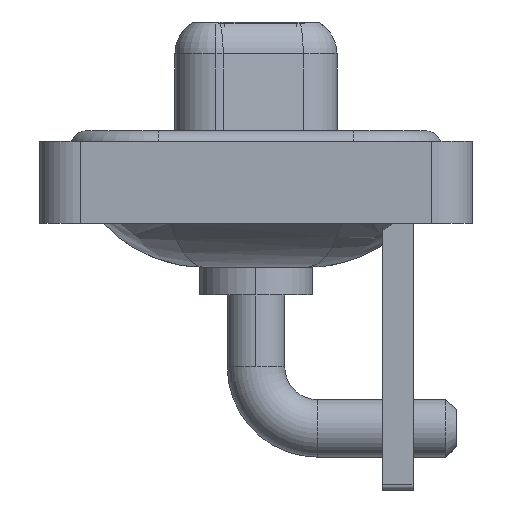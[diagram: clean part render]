
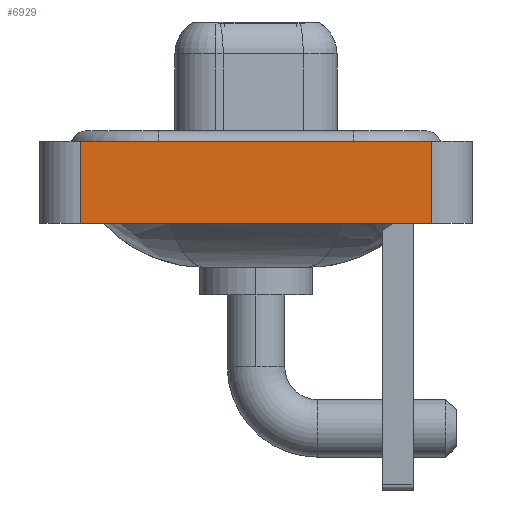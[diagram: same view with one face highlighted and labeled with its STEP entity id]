
A CAD part, left-side view. The second image highlights one B-rep face of the part: STEP entity #6929.
In plain terms, the highlighted planar face has unit normal (-1, 0, 0).
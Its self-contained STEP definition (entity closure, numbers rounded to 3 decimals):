
#339 = PLANE ( 'NONE',  #5335 ) ;
#2868 = DIRECTION ( 'NONE',  ( 0., -1., 0. ) ) ;
#2964 = DIRECTION ( 'NONE',  ( -1., 0., 0. ) ) ;
#3488 = EDGE_CURVE ( 'NONE', #15932, #4345, #7195, .T. ) ;
#4280 = DIRECTION ( 'NONE',  ( 0., 0., 1. ) ) ;
#4345 = VERTEX_POINT ( 'NONE', #6886 ) ;
#5335 = AXIS2_PLACEMENT_3D ( 'NONE', #16402, #2964, #4280 ) ;
#5343 = EDGE_CURVE ( 'NONE', #10010, #9417, #14915, .T. ) ;
#5426 = VECTOR ( 'NONE', #7169, 1000. ) ;
#5608 = CARTESIAN_POINT ( 'NONE',  ( -7.35, -8.55, 0.4 ) ) ;
#6595 = VECTOR ( 'NONE', #15816, 1000. ) ;
#6681 = LINE ( 'NONE', #10476, #6595 ) ;
#6766 = CARTESIAN_POINT ( 'NONE',  ( -7.35, 8.55, -3.6 ) ) ;
#6886 = CARTESIAN_POINT ( 'NONE',  ( -7.35, -8.55, 0.4 ) ) ;
#6903 = LINE ( 'NONE', #10872, #5426 ) ;
#6929 = ADVANCED_FACE ( 'NONE', ( #8513 ), #339, .T. ) ;
#7169 = DIRECTION ( 'NONE',  ( 0., 0., 1. ) ) ;
#7195 = LINE ( 'NONE', #5608, #8643 ) ;
#7876 = ORIENTED_EDGE ( 'NONE', *, *, #8765, .F. ) ;
#8371 = EDGE_LOOP ( 'NONE', ( #15508, #9487, #7876, #15078 ) ) ;
#8513 = FACE_OUTER_BOUND ( 'NONE', #8371, .T. ) ;
#8643 = VECTOR ( 'NONE', #12220, 1000. ) ;
#8765 = EDGE_CURVE ( 'NONE', #10010, #15932, #6903, .T. ) ;
#8960 = CARTESIAN_POINT ( 'NONE',  ( -7.35, -8.55, -3.6 ) ) ;
#9417 = VERTEX_POINT ( 'NONE', #8960 ) ;
#9487 = ORIENTED_EDGE ( 'NONE', *, *, #3488, .F. ) ;
#10010 = VERTEX_POINT ( 'NONE', #6766 ) ;
#10104 = EDGE_CURVE ( 'NONE', #9417, #4345, #6681, .T. ) ;
#10476 = CARTESIAN_POINT ( 'NONE',  ( -7.35, -8.55, -3.6 ) ) ;
#10872 = CARTESIAN_POINT ( 'NONE',  ( -7.35, 8.55, -3.6 ) ) ;
#12220 = DIRECTION ( 'NONE',  ( 0., -1., 0. ) ) ;
#12283 = CARTESIAN_POINT ( 'NONE',  ( -7.35, -8.55, -3.6 ) ) ;
#14404 = CARTESIAN_POINT ( 'NONE',  ( -7.35, 8.55, 0.4 ) ) ;
#14915 = LINE ( 'NONE', #12283, #15708 ) ;
#15078 = ORIENTED_EDGE ( 'NONE', *, *, #5343, .T. ) ;
#15508 = ORIENTED_EDGE ( 'NONE', *, *, #10104, .T. ) ;
#15708 = VECTOR ( 'NONE', #2868, 1000. ) ;
#15816 = DIRECTION ( 'NONE',  ( 0., 0., 1. ) ) ;
#15932 = VERTEX_POINT ( 'NONE', #14404 ) ;
#16402 = CARTESIAN_POINT ( 'NONE',  ( -7.35, -8.55, -3.6 ) ) ;
